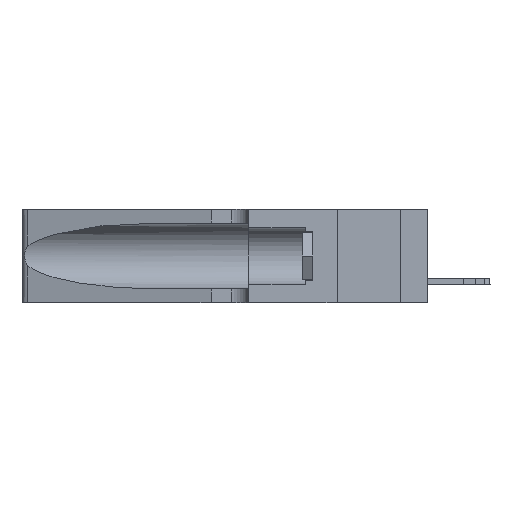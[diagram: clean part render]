
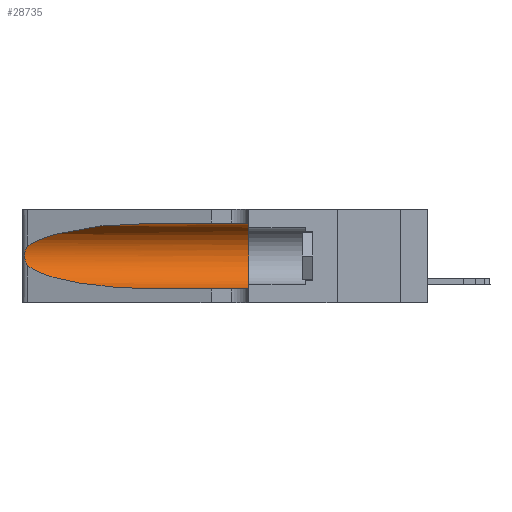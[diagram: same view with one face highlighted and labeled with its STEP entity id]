
A CAD part, left-side view. The second image highlights one B-rep face of the part: STEP entity #28735.
In plain terms, the highlighted cylindrical face has radius 3.308 mm (diameter 6.617 mm), a partial arc.
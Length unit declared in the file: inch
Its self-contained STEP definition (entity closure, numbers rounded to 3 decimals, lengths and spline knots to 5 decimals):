
#864 = VECTOR ( 'NONE', #15196, 39.37008 ) ;
#1087 = DIRECTION ( 'NONE',  ( 0., 0., -1. ) ) ;
#1623 = CARTESIAN_POINT ( 'NONE',  ( 0.25487, 1.22718, 0.22369 ) ) ;
#1888 = CARTESIAN_POINT ( 'NONE',  ( 0.25854, 1.2359, 0.20912 ) ) ;
#2290 = VERTEX_POINT ( 'NONE', #26007 ) ;
#3319 = CARTESIAN_POINT ( 'NONE',  ( 0.1305, 0.72297, 0.31525 ) ) ;
#3400 = LINE ( 'NONE', #17270, #11339 ) ;
#5237 = EDGE_LOOP ( 'NONE', ( #26752, #28952, #17290, #26883, #9836, #19704 ) ) ;
#5589 = DIRECTION ( 'NONE',  ( 0., -1., 0. ) ) ;
#6407 = AXIS2_PLACEMENT_3D ( 'NONE', #31297, #14296, #24100 ) ;
#6478 = CYLINDRICAL_SURFACE ( 'NONE', #13148, 0.13025 ) ;
#6590 = CARTESIAN_POINT ( 'NONE',  ( 0.26018, 1.23835, 0.19895 ) ) ;
#9167 = CARTESIAN_POINT ( 'NONE',  ( 0.26075, 1.23896, 0.178 ) ) ;
#9206 = CARTESIAN_POINT ( 'NONE',  ( 0.25487, 1.22718, 0.14631 ) ) ;
#9836 = ORIENTED_EDGE ( 'NONE', *, *, #29880, .F. ) ;
#11339 = VECTOR ( 'NONE', #5589, 39.37008 ) ;
#11449 = EDGE_CURVE ( 'NONE', #21280, #19202, #24034, .T. ) ;
#11674 = EDGE_CURVE ( 'NONE', #19202, #31189, #21282, .T. ) ;
#11929 = EDGE_CURVE ( 'NONE', #15145, #19421, #20094, .T. ) ;
#12946 = DIRECTION ( 'NONE',  ( 0., -1., 0. ) ) ;
#13148 = AXIS2_PLACEMENT_3D ( 'NONE', #20845, #12946, #1087 ) ;
#13271 = CARTESIAN_POINT ( 'NONE',  ( 0.2373, 1.15595, 0.28018 ) ) ;
#13624 = CARTESIAN_POINT ( 'NONE',  ( 0.25789, 1.23486, 0.15765 ) ) ;
#14296 = DIRECTION ( 'NONE',  ( 0., 1., 0. ) ) ;
#15145 = VERTEX_POINT ( 'NONE', #22653 ) ;
#15196 = DIRECTION ( 'NONE',  ( 0., -1., 0. ) ) ;
#16107 = CARTESIAN_POINT ( 'NONE',  ( 0.25487, 1.22718, 0.22369 ) ) ;
#16329 = CARTESIAN_POINT ( 'NONE',  ( 0.25787, 1.23484, 0.2124 ) ) ;
#17270 = CARTESIAN_POINT ( 'NONE',  ( 0.1305, 1.61858, 0.31525 ) ) ;
#17290 = ORIENTED_EDGE ( 'NONE', *, *, #30500, .T. ) ;
#17390 = FACE_OUTER_BOUND ( 'NONE', #5237, .T. ) ;
#17457 = CARTESIAN_POINT ( 'NONE',  ( 0.1305, 1.61858, 0.05475 ) ) ;
#18252 = CARTESIAN_POINT ( 'NONE',  ( 0.18966, 0.96281, 0.31525 ) ) ;
#18348 = CARTESIAN_POINT ( 'NONE',  ( 0.1305, 0.72297, 0.31525 ) ) ;
#19202 = VERTEX_POINT ( 'NONE', #16107 ) ;
#19319 = CARTESIAN_POINT ( 'NONE',  ( 0.25555, 1.22993, 0.14849 ) ) ;
#19385 = CARTESIAN_POINT ( 'NONE',  ( 0.18966, 0.96281, 0.05475 ) ) ;
#19421 = VERTEX_POINT ( 'NONE', #28928 ) ;
#19704 = ORIENTED_EDGE ( 'NONE', *, *, #20316, .F. ) ;
#20094 = LINE ( 'NONE', #17457, #864 ) ;
#20316 = EDGE_CURVE ( 'NONE', #21280, #2290, #3400, .T. ) ;
#20845 = CARTESIAN_POINT ( 'NONE',  ( 0.1305, 1.61858, 0.185 ) ) ;
#20938 = CARTESIAN_POINT ( 'NONE',  ( 0.25555, 1.22994, 0.2215 ) ) ;
#21047 = CARTESIAN_POINT ( 'NONE',  ( 0.25639, 1.23184, 0.21858 ) ) ;
#21280 = VERTEX_POINT ( 'NONE', #3319 ) ;
#21282 = B_SPLINE_CURVE_WITH_KNOTS ( 'NONE', 3,
 ( #28270, #20938, #21047, #16329, #1888, #6590, #25759, #9167, #25657, #28051, #13624, #30493, #19319, #26659 ),
 .UNSPECIFIED., .F., .F.,
 ( 4, 2, 2, 2, 2, 2, 4 ),
 ( 0., 0.00027, 0.00053, 0.00107, 0.0016, 0.00187, 0.00214 ),
 .UNSPECIFIED. ) ;
#21833 = CARTESIAN_POINT ( 'NONE',  ( 0.1305, 0.72297, 0.05475 ) ) ;
#22653 = CARTESIAN_POINT ( 'NONE',  ( 0.1305, 0.72297, 0.05475 ) ) ;
#24034 =( BOUNDED_CURVE ( )  B_SPLINE_CURVE ( 3, ( #18348, #18252, #13271, #1623 ),
 .UNSPECIFIED., .F., .F. ) 
 B_SPLINE_CURVE_WITH_KNOTS ( ( 4, 4 ),
 ( 1.5708, 2.84003 ),
 .UNSPECIFIED. ) 
 CURVE ( )  GEOMETRIC_REPRESENTATION_ITEM ( )  RATIONAL_B_SPLINE_CURVE ( ( 1., 0.87, 0.87, 1. ) ) 
 REPRESENTATION_ITEM ( '' )  );
#24100 = DIRECTION ( 'NONE',  ( 0., 0., 1. ) ) ;
#25657 = CARTESIAN_POINT ( 'NONE',  ( 0.26017, 1.23833, 0.17102 ) ) ;
#25759 = CARTESIAN_POINT ( 'NONE',  ( 0.26075, 1.23896, 0.19203 ) ) ;
#25978 =( BOUNDED_CURVE ( )  B_SPLINE_CURVE ( 3, ( #9206, #28647, #19385, #21833 ),
 .UNSPECIFIED., .F., .F. ) 
 B_SPLINE_CURVE_WITH_KNOTS ( ( 4, 4 ),
 ( 3.44316, 4.71239 ),
 .UNSPECIFIED. ) 
 CURVE ( )  GEOMETRIC_REPRESENTATION_ITEM ( )  RATIONAL_B_SPLINE_CURVE ( ( 1., 0.87, 0.87, 1. ) ) 
 REPRESENTATION_ITEM ( '' )  );
#26007 = CARTESIAN_POINT ( 'NONE',  ( 0.1305, 0.35, 0.31525 ) ) ;
#26659 = CARTESIAN_POINT ( 'NONE',  ( 0.25487, 1.22718, 0.14631 ) ) ;
#26752 = ORIENTED_EDGE ( 'NONE', *, *, #11449, .T. ) ;
#26883 = ORIENTED_EDGE ( 'NONE', *, *, #11929, .T. ) ;
#28051 = CARTESIAN_POINT ( 'NONE',  ( 0.25856, 1.23593, 0.16098 ) ) ;
#28270 = CARTESIAN_POINT ( 'NONE',  ( 0.25487, 1.22718, 0.22369 ) ) ;
#28647 = CARTESIAN_POINT ( 'NONE',  ( 0.2373, 1.15595, 0.08982 ) ) ;
#28735 = ADVANCED_FACE ( 'NONE', ( #17390 ), #6478, .F. ) ;
#28781 = CIRCLE ( 'NONE', #6407, 0.13025 ) ;
#28928 = CARTESIAN_POINT ( 'NONE',  ( 0.1305, 0.35, 0.05475 ) ) ;
#28952 = ORIENTED_EDGE ( 'NONE', *, *, #11674, .T. ) ;
#29337 = CARTESIAN_POINT ( 'NONE',  ( 0.25487, 1.22718, 0.14631 ) ) ;
#29880 = EDGE_CURVE ( 'NONE', #2290, #19421, #28781, .T. ) ;
#30493 = CARTESIAN_POINT ( 'NONE',  ( 0.25639, 1.23186, 0.15144 ) ) ;
#30500 = EDGE_CURVE ( 'NONE', #31189, #15145, #25978, .T. ) ;
#31189 = VERTEX_POINT ( 'NONE', #29337 ) ;
#31297 = CARTESIAN_POINT ( 'NONE',  ( 0.1305, 0.35, 0.185 ) ) ;
